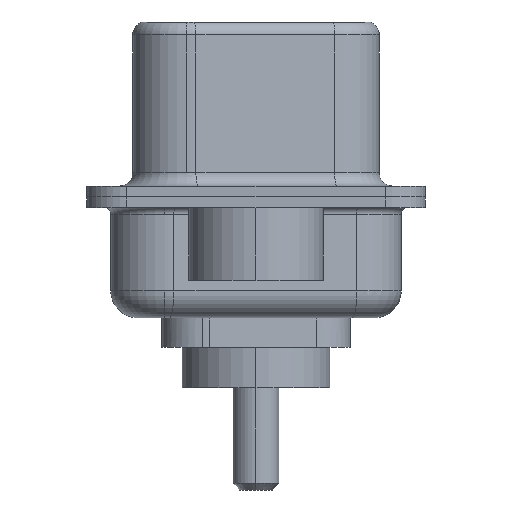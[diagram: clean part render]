
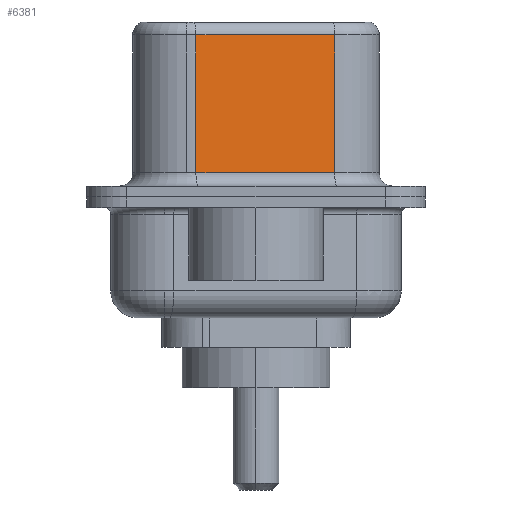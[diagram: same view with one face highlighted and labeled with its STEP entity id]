
A CAD part, left-side view. The second image highlights one B-rep face of the part: STEP entity #6381.
In plain terms, the highlighted planar face has unit normal (-0.985, -0.174, 0).
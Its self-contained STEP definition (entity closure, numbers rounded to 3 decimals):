
#261 = VECTOR ( 'NONE', #5595, 1000. ) ;
#904 = ORIENTED_EDGE ( 'NONE', *, *, #13956, .T. ) ;
#935 = EDGE_LOOP ( 'NONE', ( #13342, #904, #1343, #4873 ) ) ;
#1104 = CARTESIAN_POINT ( 'NONE',  ( 4.58, -2.927, 6.52 ) ) ;
#1343 = ORIENTED_EDGE ( 'NONE', *, *, #15651, .T. ) ;
#1905 = VERTEX_POINT ( 'NONE', #3379 ) ;
#2706 = LINE ( 'NONE', #8798, #12685 ) ;
#2906 = VECTOR ( 'NONE', #3613, 1000. ) ;
#2960 = CARTESIAN_POINT ( 'NONE',  ( 4.58, -2.927, 0.9 ) ) ;
#3192 = DIRECTION ( 'NONE',  ( 0., 0., -1. ) ) ;
#3239 = VERTEX_POINT ( 'NONE', #6471 ) ;
#3343 = CARTESIAN_POINT ( 'NONE',  ( 4.58, -2.927, 0.9 ) ) ;
#3379 = CARTESIAN_POINT ( 'NONE',  ( 4.58, -2.927, 6.02 ) ) ;
#3392 = AXIS2_PLACEMENT_3D ( 'NONE', #4634, #12463, #4678 ) ;
#3613 = DIRECTION ( 'NONE',  ( 0., 0., -1. ) ) ;
#4634 = CARTESIAN_POINT ( 'NONE',  ( 4.58, -2.927, 6.52 ) ) ;
#4678 = DIRECTION ( 'NONE',  ( -0.174, 0.985, 0. ) ) ;
#4842 = DIRECTION ( 'NONE',  ( -0.174, 0.985, 0. ) ) ;
#4873 = ORIENTED_EDGE ( 'NONE', *, *, #10472, .T. ) ;
#5595 = DIRECTION ( 'NONE',  ( 0.174, -0.985, 0. ) ) ;
#5773 = EDGE_CURVE ( 'NONE', #1905, #9581, #13250, .T. ) ;
#6381 = ADVANCED_FACE ( 'NONE', ( #11114 ), #15000, .F. ) ;
#6471 = CARTESIAN_POINT ( 'NONE',  ( 3.67, 2.233, 6.02 ) ) ;
#6755 = CARTESIAN_POINT ( 'NONE',  ( 3.67, 2.233, 0.9 ) ) ;
#8656 = VERTEX_POINT ( 'NONE', #6755 ) ;
#8798 = CARTESIAN_POINT ( 'NONE',  ( 4.58, -2.927, 6.02 ) ) ;
#9581 = VERTEX_POINT ( 'NONE', #3343 ) ;
#10142 = LINE ( 'NONE', #13486, #13457 ) ;
#10472 = EDGE_CURVE ( 'NONE', #8656, #9581, #16431, .T. ) ;
#11114 = FACE_OUTER_BOUND ( 'NONE', #935, .T. ) ;
#12463 = DIRECTION ( 'NONE',  ( 0.985, 0.174, 0. ) ) ;
#12685 = VECTOR ( 'NONE', #4842, 1000. ) ;
#13250 = LINE ( 'NONE', #1104, #2906 ) ;
#13342 = ORIENTED_EDGE ( 'NONE', *, *, #5773, .F. ) ;
#13457 = VECTOR ( 'NONE', #3192, 1000. ) ;
#13486 = CARTESIAN_POINT ( 'NONE',  ( 3.67, 2.233, 6.52 ) ) ;
#13956 = EDGE_CURVE ( 'NONE', #1905, #3239, #2706, .T. ) ;
#15000 = PLANE ( 'NONE',  #3392 ) ;
#15651 = EDGE_CURVE ( 'NONE', #3239, #8656, #10142, .T. ) ;
#16431 = LINE ( 'NONE', #2960, #261 ) ;
